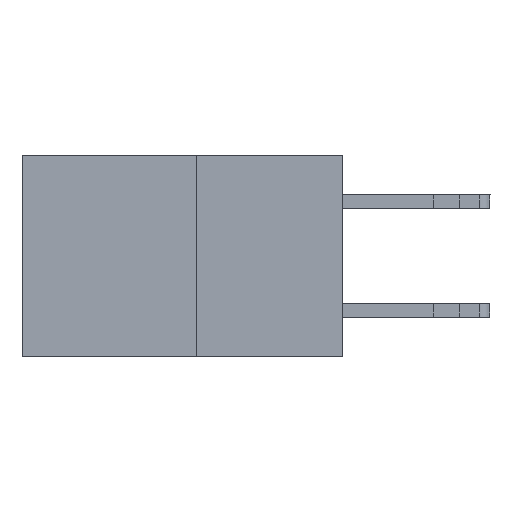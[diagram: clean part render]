
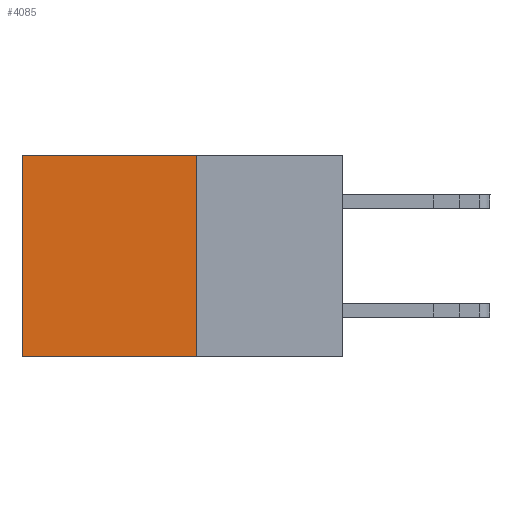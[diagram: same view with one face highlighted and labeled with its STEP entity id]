
A CAD part, left-side view. The second image highlights one B-rep face of the part: STEP entity #4085.
In plain terms, the highlighted planar face has unit normal (-1, 0, 0).
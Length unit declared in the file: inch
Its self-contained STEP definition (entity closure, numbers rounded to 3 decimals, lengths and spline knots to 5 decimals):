
#98 = LINE ( 'NONE', #10523, #6378 ) ;
#831 = CARTESIAN_POINT ( 'NONE',  ( 0.277, 0.27, -0.37 ) ) ;
#1085 = ORIENTED_EDGE ( 'NONE', *, *, #7909, .F. ) ;
#1327 = ORIENTED_EDGE ( 'NONE', *, *, #12572, .T. ) ;
#1418 = VECTOR ( 'NONE', #3474, 39.37008 ) ;
#1889 = CARTESIAN_POINT ( 'NONE',  ( 0.277, 0.59, -0.37 ) ) ;
#1908 = VERTEX_POINT ( 'NONE', #1889 ) ;
#1920 = DIRECTION ( 'NONE',  ( 1., 0., 0. ) ) ;
#1990 = DIRECTION ( 'NONE',  ( 0., 0., -1. ) ) ;
#2284 = LINE ( 'NONE', #5217, #5451 ) ;
#2529 = DIRECTION ( 'NONE',  ( 0., 0., -1. ) ) ;
#2663 = EDGE_CURVE ( 'NONE', #3884, #5519, #3161, .T. ) ;
#2761 = CARTESIAN_POINT ( 'NONE',  ( 0.277, 0.27, 0. ) ) ;
#3161 = LINE ( 'NONE', #12820, #1418 ) ;
#3474 = DIRECTION ( 'NONE',  ( 0., 0., -1. ) ) ;
#3884 = VERTEX_POINT ( 'NONE', #2761 ) ;
#4085 = ADVANCED_FACE ( 'NONE', ( #6905 ), #7988, .F. ) ;
#4266 = DIRECTION ( 'NONE',  ( 0., 1., 0. ) ) ;
#4981 = CARTESIAN_POINT ( 'NONE',  ( 0.277, 0.59, 0. ) ) ;
#5217 = CARTESIAN_POINT ( 'NONE',  ( 0.277, 0.27, 0. ) ) ;
#5451 = VECTOR ( 'NONE', #9435, 39.37008 ) ;
#5519 = VERTEX_POINT ( 'NONE', #8128 ) ;
#5810 = LINE ( 'NONE', #8789, #11723 ) ;
#5819 = EDGE_CURVE ( 'NONE', #6833, #1908, #5810, .T. ) ;
#6378 = VECTOR ( 'NONE', #4266, 39.37008 ) ;
#6600 = ORIENTED_EDGE ( 'NONE', *, *, #2663, .F. ) ;
#6788 = AXIS2_PLACEMENT_3D ( 'NONE', #831, #1920, #1990 ) ;
#6833 = VERTEX_POINT ( 'NONE', #4981 ) ;
#6905 = FACE_OUTER_BOUND ( 'NONE', #13121, .T. ) ;
#7909 = EDGE_CURVE ( 'NONE', #5519, #1908, #98, .T. ) ;
#7988 = PLANE ( 'NONE',  #6788 ) ;
#8128 = CARTESIAN_POINT ( 'NONE',  ( 0.277, 0.27, -0.37 ) ) ;
#8789 = CARTESIAN_POINT ( 'NONE',  ( 0.277, 0.59, -0.37 ) ) ;
#9435 = DIRECTION ( 'NONE',  ( 0., 1., 0. ) ) ;
#10523 = CARTESIAN_POINT ( 'NONE',  ( 0.277, 0.27, -0.37 ) ) ;
#11723 = VECTOR ( 'NONE', #2529, 39.37008 ) ;
#12341 = ORIENTED_EDGE ( 'NONE', *, *, #5819, .T. ) ;
#12572 = EDGE_CURVE ( 'NONE', #3884, #6833, #2284, .T. ) ;
#12820 = CARTESIAN_POINT ( 'NONE',  ( 0.277, 0.27, -0.37 ) ) ;
#13121 = EDGE_LOOP ( 'NONE', ( #12341, #1085, #6600, #1327 ) ) ;
